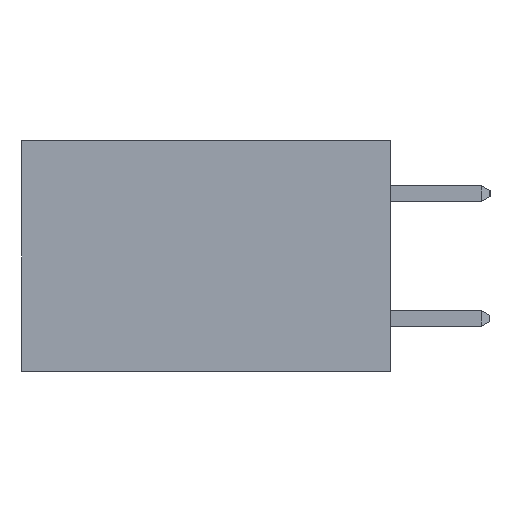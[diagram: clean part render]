
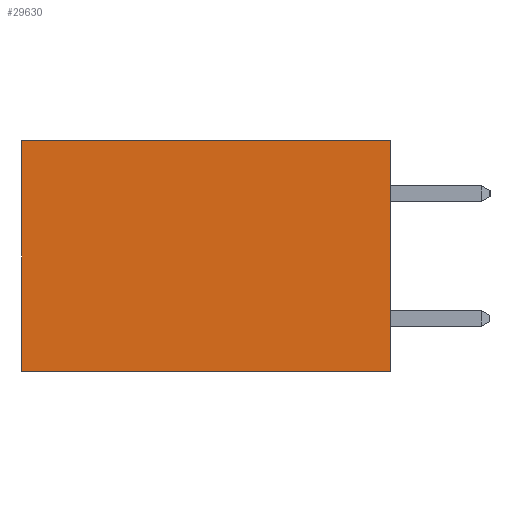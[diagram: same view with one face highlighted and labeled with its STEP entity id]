
A CAD part, left-side view. The second image highlights one B-rep face of the part: STEP entity #29630.
In plain terms, the highlighted planar face has unit normal (-1, 0, 0).
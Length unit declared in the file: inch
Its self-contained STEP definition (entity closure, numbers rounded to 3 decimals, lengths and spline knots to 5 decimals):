
#198 = EDGE_CURVE ( 'NONE', #23034, #5531, #17593, .T. ) ;
#1073 = DIRECTION ( 'NONE',  ( 1., 0., 0. ) ) ;
#2597 = CARTESIAN_POINT ( 'NONE',  ( 0.277, 0.59, -0.37 ) ) ;
#2600 = ORIENTED_EDGE ( 'NONE', *, *, #21727, .F. ) ;
#2683 = ORIENTED_EDGE ( 'NONE', *, *, #9484, .T. ) ;
#4306 = LINE ( 'NONE', #20588, #16652 ) ;
#4600 = VERTEX_POINT ( 'NONE', #11485 ) ;
#5531 = VERTEX_POINT ( 'NONE', #20676 ) ;
#6167 = VECTOR ( 'NONE', #21569, 39.37008 ) ;
#7204 = VECTOR ( 'NONE', #25587, 39.37008 ) ;
#7733 = PLANE ( 'NONE',  #13503 ) ;
#7907 = LINE ( 'NONE', #2597, #7204 ) ;
#9484 = EDGE_CURVE ( 'NONE', #23034, #27110, #4306, .T. ) ;
#9858 = CARTESIAN_POINT ( 'NONE',  ( 0.277, 0., -0.37 ) ) ;
#10596 = VECTOR ( 'NONE', #16244, 39.37008 ) ;
#11485 = CARTESIAN_POINT ( 'NONE',  ( 0.277, 0.59, -0.37 ) ) ;
#12793 = CARTESIAN_POINT ( 'NONE',  ( 0.277, 0.59, 0. ) ) ;
#13503 = AXIS2_PLACEMENT_3D ( 'NONE', #21783, #1073, #17250 ) ;
#13655 = DIRECTION ( 'NONE',  ( 0., 1., 0. ) ) ;
#15392 = FACE_OUTER_BOUND ( 'NONE', #16721, .T. ) ;
#15830 = CARTESIAN_POINT ( 'NONE',  ( 0.277, 0., -0.37 ) ) ;
#16244 = DIRECTION ( 'NONE',  ( 0., 0., -1. ) ) ;
#16652 = VECTOR ( 'NONE', #13655, 39.37008 ) ;
#16721 = EDGE_LOOP ( 'NONE', ( #23105, #2600, #17116, #2683 ) ) ;
#16885 = EDGE_CURVE ( 'NONE', #27110, #4600, #7907, .T. ) ;
#17116 = ORIENTED_EDGE ( 'NONE', *, *, #198, .F. ) ;
#17250 = DIRECTION ( 'NONE',  ( 0., 0., -1. ) ) ;
#17593 = LINE ( 'NONE', #15830, #10596 ) ;
#18912 = CARTESIAN_POINT ( 'NONE',  ( 0.277, 0., 0. ) ) ;
#20588 = CARTESIAN_POINT ( 'NONE',  ( 0.277, 0., 0. ) ) ;
#20676 = CARTESIAN_POINT ( 'NONE',  ( 0.277, 0., -0.37 ) ) ;
#21569 = DIRECTION ( 'NONE',  ( 0., 1., 0. ) ) ;
#21727 = EDGE_CURVE ( 'NONE', #5531, #4600, #25366, .T. ) ;
#21783 = CARTESIAN_POINT ( 'NONE',  ( 0.277, 0., -0.37 ) ) ;
#23034 = VERTEX_POINT ( 'NONE', #18912 ) ;
#23105 = ORIENTED_EDGE ( 'NONE', *, *, #16885, .T. ) ;
#25366 = LINE ( 'NONE', #9858, #6167 ) ;
#25587 = DIRECTION ( 'NONE',  ( 0., 0., -1. ) ) ;
#27110 = VERTEX_POINT ( 'NONE', #12793 ) ;
#29630 = ADVANCED_FACE ( 'NONE', ( #15392 ), #7733, .F. ) ;
